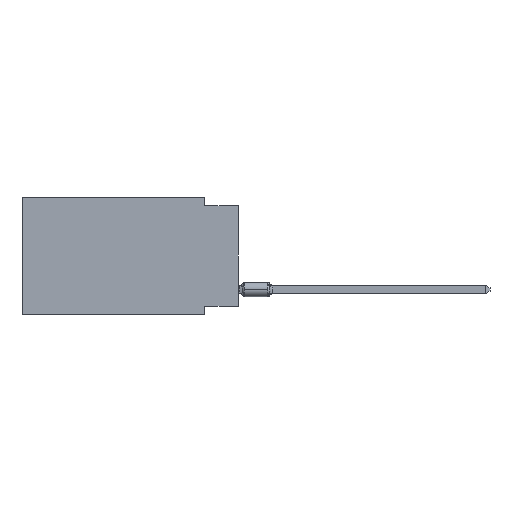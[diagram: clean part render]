
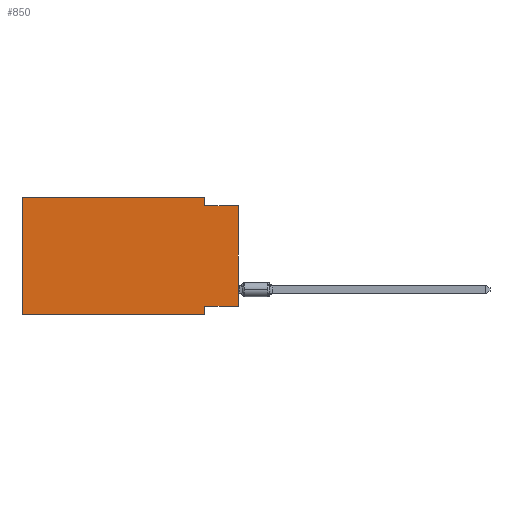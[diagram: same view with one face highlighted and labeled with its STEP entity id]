
A CAD part, left-side view. The second image highlights one B-rep face of the part: STEP entity #850.
In plain terms, the highlighted planar face has unit normal (-1, 0, 0).
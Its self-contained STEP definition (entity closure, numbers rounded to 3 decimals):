
#145 = CARTESIAN_POINT ( 'NONE',  ( 0., 2.54, -8.255 ) ) ;
#850 = ADVANCED_FACE ( 'NONE', ( #1704 ), #10542, .F. ) ;
#1588 = ORIENTED_EDGE ( 'NONE', *, *, #9274, .F. ) ;
#1622 = ORIENTED_EDGE ( 'NONE', *, *, #2828, .F. ) ;
#1704 = FACE_OUTER_BOUND ( 'NONE', #1804, .T. ) ;
#1740 = EDGE_CURVE ( 'NONE', #3943, #14022, #3458, .T. ) ;
#1804 = EDGE_LOOP ( 'NONE', ( #5671, #12773, #13144, #1622, #5794, #2988, #1588, #8884 ) ) ;
#1840 = VECTOR ( 'NONE', #7964, 1000. ) ;
#2124 = VERTEX_POINT ( 'NONE', #4909 ) ;
#2317 = VERTEX_POINT ( 'NONE', #8864 ) ;
#2828 = EDGE_CURVE ( 'NONE', #14022, #13645, #10912, .T. ) ;
#2988 = ORIENTED_EDGE ( 'NONE', *, *, #9767, .T. ) ;
#3059 = VECTOR ( 'NONE', #6286, 1000. ) ;
#3158 = CARTESIAN_POINT ( 'NONE',  ( 0., 2.54, 0. ) ) ;
#3458 = LINE ( 'NONE', #5213, #1840 ) ;
#3528 = CARTESIAN_POINT ( 'NONE',  ( 0., 0., -8.255 ) ) ;
#3943 = VERTEX_POINT ( 'NONE', #19060 ) ;
#4512 = VECTOR ( 'NONE', #16887, 1000. ) ;
#4580 = CARTESIAN_POINT ( 'NONE',  ( 0., 2.54, 0. ) ) ;
#4909 = CARTESIAN_POINT ( 'NONE',  ( 0., 0., -0.635 ) ) ;
#5065 = DIRECTION ( 'NONE',  ( 0., -1., 0. ) ) ;
#5213 = CARTESIAN_POINT ( 'NONE',  ( 0., 16.383, 0. ) ) ;
#5671 = ORIENTED_EDGE ( 'NONE', *, *, #10463, .T. ) ;
#5794 = ORIENTED_EDGE ( 'NONE', *, *, #1740, .F. ) ;
#6049 = CARTESIAN_POINT ( 'NONE',  ( 0., 0., -8.255 ) ) ;
#6183 = CARTESIAN_POINT ( 'NONE',  ( 0., 2.54, -0.635 ) ) ;
#6254 = LINE ( 'NONE', #6439, #7691 ) ;
#6286 = DIRECTION ( 'NONE',  ( 0., 1., 0. ) ) ;
#6339 = LINE ( 'NONE', #16426, #14847 ) ;
#6439 = CARTESIAN_POINT ( 'NONE',  ( 0., 0., 0. ) ) ;
#6767 = CARTESIAN_POINT ( 'NONE',  ( 0., 16.383, -8.89 ) ) ;
#7449 = VERTEX_POINT ( 'NONE', #145 ) ;
#7597 = CARTESIAN_POINT ( 'NONE',  ( 0., 16.383, 0. ) ) ;
#7691 = VECTOR ( 'NONE', #16537, 1000. ) ;
#7697 = DIRECTION ( 'NONE',  ( 1., 0., 0. ) ) ;
#7964 = DIRECTION ( 'NONE',  ( 0., 0., 1. ) ) ;
#7965 = DIRECTION ( 'NONE',  ( 0., 0., -1. ) ) ;
#8864 = CARTESIAN_POINT ( 'NONE',  ( 0., 2.54, -8.89 ) ) ;
#8884 = ORIENTED_EDGE ( 'NONE', *, *, #16113, .F. ) ;
#9274 = EDGE_CURVE ( 'NONE', #7449, #2317, #6339, .T. ) ;
#9473 = CARTESIAN_POINT ( 'NONE',  ( 0., 0., -0.635 ) ) ;
#9767 = EDGE_CURVE ( 'NONE', #3943, #2317, #9898, .T. ) ;
#9898 = LINE ( 'NONE', #6767, #14530 ) ;
#10074 = DIRECTION ( 'NONE',  ( 0., -1., 0. ) ) ;
#10463 = EDGE_CURVE ( 'NONE', #13641, #2124, #6254, .T. ) ;
#10542 = PLANE ( 'NONE',  #16828 ) ;
#10912 = LINE ( 'NONE', #11978, #4512 ) ;
#11659 = EDGE_CURVE ( 'NONE', #14909, #2124, #18195, .T. ) ;
#11978 = CARTESIAN_POINT ( 'NONE',  ( 0., 16.383, 0. ) ) ;
#12773 = ORIENTED_EDGE ( 'NONE', *, *, #11659, .F. ) ;
#13144 = ORIENTED_EDGE ( 'NONE', *, *, #14565, .F. ) ;
#13641 = VERTEX_POINT ( 'NONE', #6049 ) ;
#13645 = VERTEX_POINT ( 'NONE', #4580 ) ;
#13883 = DIRECTION ( 'NONE',  ( 0., 0., -1. ) ) ;
#13946 = LINE ( 'NONE', #3158, #17980 ) ;
#14022 = VERTEX_POINT ( 'NONE', #19350 ) ;
#14530 = VECTOR ( 'NONE', #10074, 1000. ) ;
#14565 = EDGE_CURVE ( 'NONE', #13645, #14909, #13946, .T. ) ;
#14847 = VECTOR ( 'NONE', #13883, 1000. ) ;
#14909 = VERTEX_POINT ( 'NONE', #6183 ) ;
#16113 = EDGE_CURVE ( 'NONE', #13641, #7449, #16762, .T. ) ;
#16426 = CARTESIAN_POINT ( 'NONE',  ( 0., 2.54, -8.89 ) ) ;
#16537 = DIRECTION ( 'NONE',  ( 0., 0., 1. ) ) ;
#16762 = LINE ( 'NONE', #3528, #3059 ) ;
#16828 = AXIS2_PLACEMENT_3D ( 'NONE', #7597, #7697, #18267 ) ;
#16887 = DIRECTION ( 'NONE',  ( 0., -1., 0. ) ) ;
#17164 = VECTOR ( 'NONE', #5065, 1000. ) ;
#17980 = VECTOR ( 'NONE', #7965, 1000. ) ;
#18195 = LINE ( 'NONE', #9473, #17164 ) ;
#18267 = DIRECTION ( 'NONE',  ( 0., 0., -1. ) ) ;
#19060 = CARTESIAN_POINT ( 'NONE',  ( 0., 16.383, -8.89 ) ) ;
#19350 = CARTESIAN_POINT ( 'NONE',  ( 0., 16.383, 0. ) ) ;
